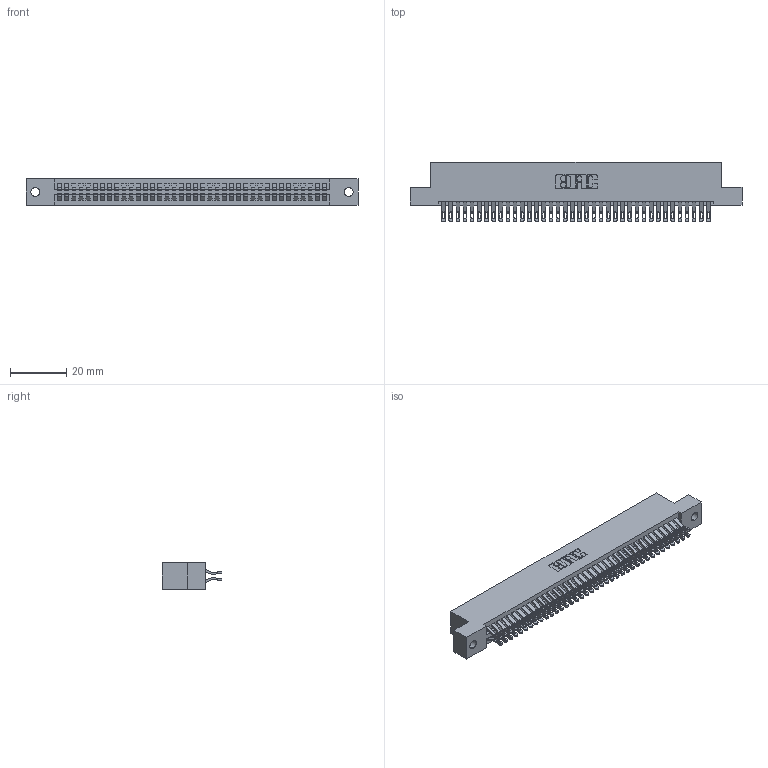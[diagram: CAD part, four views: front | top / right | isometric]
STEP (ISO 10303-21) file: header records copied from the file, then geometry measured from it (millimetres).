
FILE_DESCRIPTION (( 'STEP AP203' ), '1' );
FILE_NAME ('395-076-555-202.STEP', '2018-11-27T22:06:56', ( '' ), ( '' ), 'SwSTEP 2.0', 'SolidWorks 2016', '' );
FILE_SCHEMA (( 'CONFIG_CONTROL_DESIGN' ));
Length unit declared in the file: inch
Products named in the file (3): 345-292-001_555 Tail; 345 Part_Flush Mounting Lugs - 0.128 Dia; 395-076-555-202
Assembly tree (77 placements, depth 2):
  395-076-555-202
    345 Part_Flush Mounting Lugs - 0.128 Dia
    345-292-001_555 Tail  x76
Bounding box: 117.73 x 21.13 x 9.4 mm (x, y, z)
Volume: 11582.9 mm3; surface area: 17538.1 mm2
Topology: 77 solids, 77 shells, 4382 faces, 13793 edges, 9194 vertices
Faces by surface type: plane 2436, cylinder 1946
Entity records: 30683 total; most frequent: CARTESIAN_POINT 5182, ORIENTED_EDGE 5086, DIRECTION 4543, EDGE_CURVE 2543, LINE 2239, VECTOR 2239, VERTEX_POINT 1694, AXIS2_PLACEMENT_3D 1152
